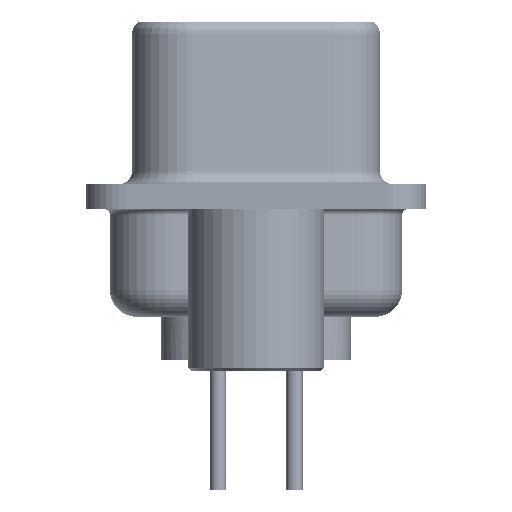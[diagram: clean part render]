
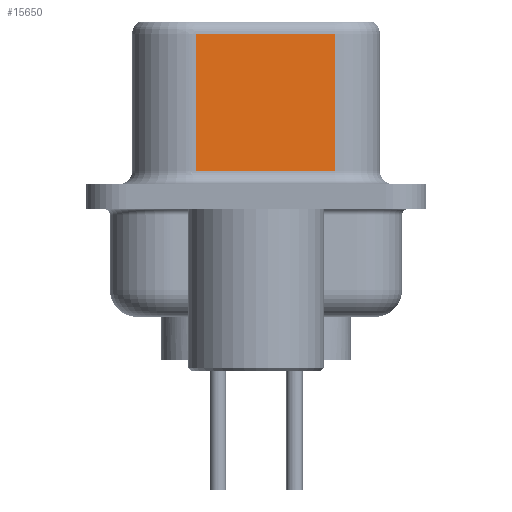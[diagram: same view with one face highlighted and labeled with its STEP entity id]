
A CAD part, left-side view. The second image highlights one B-rep face of the part: STEP entity #15650.
In plain terms, the highlighted planar face has unit normal (-0.985, -0.174, 0).
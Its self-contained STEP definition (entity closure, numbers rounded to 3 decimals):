
#578 = ORIENTED_EDGE ( 'NONE', *, *, #29217, .T. ) ;
#1987 = VECTOR ( 'NONE', #3554, 1000. ) ;
#2226 = CARTESIAN_POINT ( 'NONE',  ( 4.58, -2.927, 0.95 ) ) ;
#3167 = EDGE_CURVE ( 'NONE', #25905, #25937, #19871, .T. ) ;
#3554 = DIRECTION ( 'NONE',  ( -0.174, 0.985, 0. ) ) ;
#7862 = CARTESIAN_POINT ( 'NONE',  ( 4.58, -2.927, 0.95 ) ) ;
#7967 = CARTESIAN_POINT ( 'NONE',  ( 4.58, -2.927, 6.52 ) ) ;
#8076 = DIRECTION ( 'NONE',  ( -0.174, 0.985, 0. ) ) ;
#9057 = CARTESIAN_POINT ( 'NONE',  ( 3.67, 2.233, 6.02 ) ) ;
#9175 = EDGE_CURVE ( 'NONE', #25905, #17835, #17427, .T. ) ;
#10585 = VERTEX_POINT ( 'NONE', #10656 ) ;
#10656 = CARTESIAN_POINT ( 'NONE',  ( 3.67, 2.233, 0.95 ) ) ;
#11507 = VECTOR ( 'NONE', #29620, 1000. ) ;
#11535 = DIRECTION ( 'NONE',  ( 0.174, -0.985, 0. ) ) ;
#12331 = VECTOR ( 'NONE', #11535, 1000. ) ;
#13085 = EDGE_CURVE ( 'NONE', #17835, #10585, #20240, .T. ) ;
#15144 = CARTESIAN_POINT ( 'NONE',  ( 4.58, -2.927, 6.02 ) ) ;
#15245 = DIRECTION ( 'NONE',  ( 0.985, 0.174, 0. ) ) ;
#15371 = ORIENTED_EDGE ( 'NONE', *, *, #9175, .T. ) ;
#15392 = CARTESIAN_POINT ( 'NONE',  ( 4.58, -2.927, 6.52 ) ) ;
#15650 = ADVANCED_FACE ( 'NONE', ( #22404 ), #21799, .F. ) ;
#15653 = CARTESIAN_POINT ( 'NONE',  ( 3.67, 2.233, 6.52 ) ) ;
#17427 = LINE ( 'NONE', #15144, #1987 ) ;
#17835 = VERTEX_POINT ( 'NONE', #9057 ) ;
#18386 = AXIS2_PLACEMENT_3D ( 'NONE', #15392, #15245, #8076 ) ;
#19871 = LINE ( 'NONE', #7967, #29651 ) ;
#20240 = LINE ( 'NONE', #15653, #11507 ) ;
#21799 = PLANE ( 'NONE',  #18386 ) ;
#21873 = ORIENTED_EDGE ( 'NONE', *, *, #13085, .T. ) ;
#21895 = CARTESIAN_POINT ( 'NONE',  ( 4.58, -2.927, 6.02 ) ) ;
#22404 = FACE_OUTER_BOUND ( 'NONE', #27952, .T. ) ;
#23110 = LINE ( 'NONE', #2226, #12331 ) ;
#23959 = DIRECTION ( 'NONE',  ( 0., 0., -1. ) ) ;
#24940 = ORIENTED_EDGE ( 'NONE', *, *, #3167, .F. ) ;
#25905 = VERTEX_POINT ( 'NONE', #21895 ) ;
#25937 = VERTEX_POINT ( 'NONE', #7862 ) ;
#27952 = EDGE_LOOP ( 'NONE', ( #24940, #15371, #21873, #578 ) ) ;
#29217 = EDGE_CURVE ( 'NONE', #10585, #25937, #23110, .T. ) ;
#29620 = DIRECTION ( 'NONE',  ( 0., 0., -1. ) ) ;
#29651 = VECTOR ( 'NONE', #23959, 1000. ) ;
